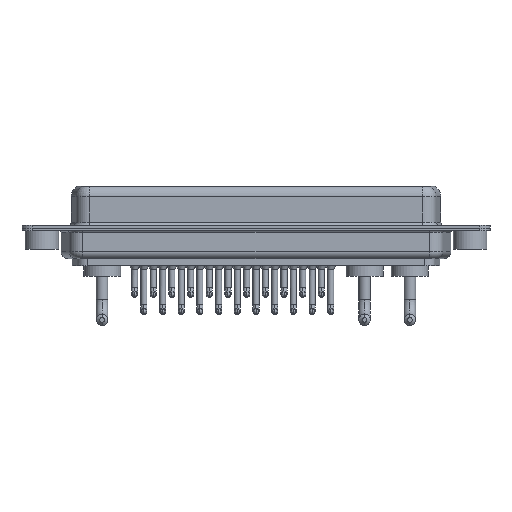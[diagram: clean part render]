
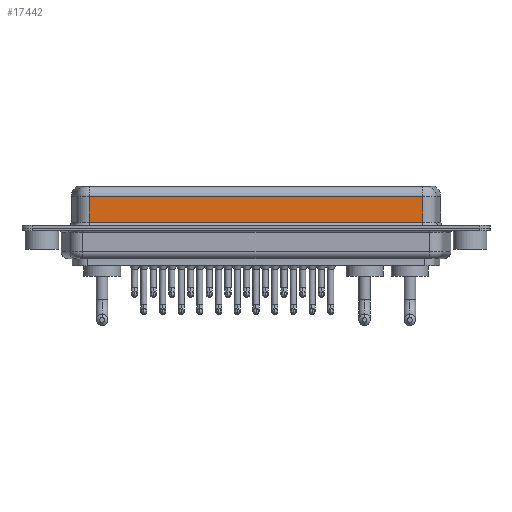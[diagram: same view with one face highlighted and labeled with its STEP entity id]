
A CAD part, front view. The second image highlights one B-rep face of the part: STEP entity #17442.
In plain terms, the highlighted planar face has unit normal (0, -1, 0).
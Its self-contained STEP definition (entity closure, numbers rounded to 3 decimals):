
#1363 = ORIENTED_EDGE ( 'NONE', *, *, #4479, .T. ) ;
#1685 = CARTESIAN_POINT ( 'NONE',  ( 56.462, -3.95, 4.65 ) ) ;
#1785 = CARTESIAN_POINT ( 'NONE',  ( 56.462, -3.95, 6.4 ) ) ;
#2127 = LINE ( 'NONE', #11526, #19815 ) ;
#3477 = CARTESIAN_POINT ( 'NONE',  ( 56.462, -3.95, 0.9 ) ) ;
#3815 = PLANE ( 'NONE',  #5507 ) ;
#4479 = EDGE_CURVE ( 'NONE', #16889, #8914, #2127, .T. ) ;
#5021 = EDGE_LOOP ( 'NONE', ( #11611, #11034, #16752, #1363 ) ) ;
#5507 = AXIS2_PLACEMENT_3D ( 'NONE', #1785, #10935, #18273 ) ;
#7094 = FACE_OUTER_BOUND ( 'NONE', #5021, .T. ) ;
#8528 = EDGE_CURVE ( 'NONE', #10692, #16889, #11933, .T. ) ;
#8830 = EDGE_CURVE ( 'NONE', #20890, #10692, #9466, .T. ) ;
#8914 = VERTEX_POINT ( 'NONE', #3477 ) ;
#9466 = LINE ( 'NONE', #18830, #19895 ) ;
#9479 = DIRECTION ( 'NONE',  ( 1., 0., 0. ) ) ;
#10692 = VERTEX_POINT ( 'NONE', #16565 ) ;
#10846 = CARTESIAN_POINT ( 'NONE',  ( 7.038, -3.95, 0.9 ) ) ;
#10935 = DIRECTION ( 'NONE',  ( 0., 1., 0. ) ) ;
#11034 = ORIENTED_EDGE ( 'NONE', *, *, #8830, .T. ) ;
#11526 = CARTESIAN_POINT ( 'NONE',  ( 56.462, -3.95, 0.9 ) ) ;
#11611 = ORIENTED_EDGE ( 'NONE', *, *, #12888, .F. ) ;
#11933 = LINE ( 'NONE', #17105, #14132 ) ;
#12685 = LINE ( 'NONE', #14751, #13482 ) ;
#12888 = EDGE_CURVE ( 'NONE', #20890, #8914, #12685, .T. ) ;
#13482 = VECTOR ( 'NONE', #14516, 1000. ) ;
#14132 = VECTOR ( 'NONE', #17466, 1000. ) ;
#14516 = DIRECTION ( 'NONE',  ( 0., 0., -1. ) ) ;
#14751 = CARTESIAN_POINT ( 'NONE',  ( 56.462, -3.95, 6.4 ) ) ;
#15007 = DIRECTION ( 'NONE',  ( -1., 0., 0. ) ) ;
#16565 = CARTESIAN_POINT ( 'NONE',  ( 7.038, -3.95, 4.65 ) ) ;
#16752 = ORIENTED_EDGE ( 'NONE', *, *, #8528, .T. ) ;
#16889 = VERTEX_POINT ( 'NONE', #10846 ) ;
#17105 = CARTESIAN_POINT ( 'NONE',  ( 7.038, -3.95, 6.4 ) ) ;
#17442 = ADVANCED_FACE ( 'NONE', ( #7094 ), #3815, .F. ) ;
#17466 = DIRECTION ( 'NONE',  ( 0., 0., -1. ) ) ;
#18273 = DIRECTION ( 'NONE',  ( 0., 0., 1. ) ) ;
#18830 = CARTESIAN_POINT ( 'NONE',  ( 56.462, -3.95, 4.65 ) ) ;
#19815 = VECTOR ( 'NONE', #9479, 1000. ) ;
#19895 = VECTOR ( 'NONE', #15007, 1000. ) ;
#20890 = VERTEX_POINT ( 'NONE', #1685 ) ;
